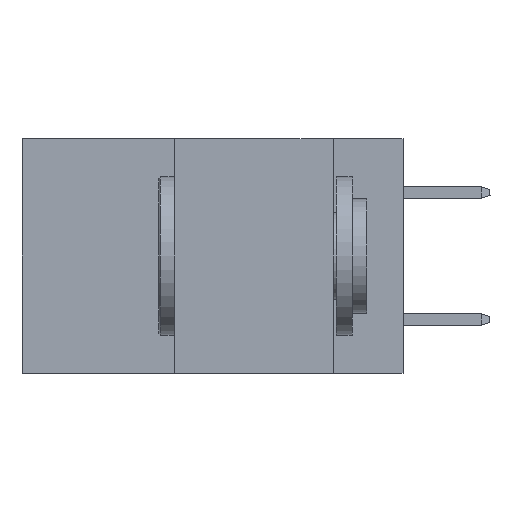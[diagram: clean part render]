
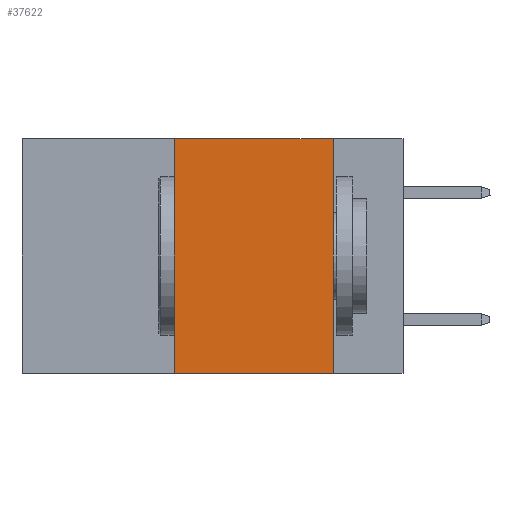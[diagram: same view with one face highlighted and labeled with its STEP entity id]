
A CAD part, left-side view. The second image highlights one B-rep face of the part: STEP entity #37622.
In plain terms, the highlighted planar face has unit normal (-1, 0, 0).
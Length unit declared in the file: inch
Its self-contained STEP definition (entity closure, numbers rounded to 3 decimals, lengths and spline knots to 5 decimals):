
#845 = DIRECTION ( 'NONE',  ( 0., -1., 0. ) ) ;
#2104 = ORIENTED_EDGE ( 'NONE', *, *, #20912, .T. ) ;
#2998 = CARTESIAN_POINT ( 'NONE',  ( 0., 0.36, 0. ) ) ;
#3638 = ORIENTED_EDGE ( 'NONE', *, *, #14503, .F. ) ;
#3734 = VERTEX_POINT ( 'NONE', #7135 ) ;
#6208 = ORIENTED_EDGE ( 'NONE', *, *, #8714, .F. ) ;
#7029 = EDGE_CURVE ( 'NONE', #15164, #10686, #27835, .T. ) ;
#7135 = CARTESIAN_POINT ( 'NONE',  ( 0., 0.36, 0. ) ) ;
#8320 = VERTEX_POINT ( 'NONE', #39944 ) ;
#8714 = EDGE_CURVE ( 'NONE', #3734, #15164, #33091, .T. ) ;
#10686 = VERTEX_POINT ( 'NONE', #17013 ) ;
#11775 = AXIS2_PLACEMENT_3D ( 'NONE', #17467, #36480, #36876 ) ;
#14037 = VECTOR ( 'NONE', #16190, 39.37008 ) ;
#14187 = VECTOR ( 'NONE', #845, 39.37008 ) ;
#14503 = EDGE_CURVE ( 'NONE', #8320, #3734, #33651, .T. ) ;
#15164 = VERTEX_POINT ( 'NONE', #24158 ) ;
#16190 = DIRECTION ( 'NONE',  ( 0., -1., 0. ) ) ;
#16596 = CARTESIAN_POINT ( 'NONE',  ( 0., 0.6, 0. ) ) ;
#16894 = VECTOR ( 'NONE', #30778, 39.37008 ) ;
#17013 = CARTESIAN_POINT ( 'NONE',  ( 0., 0.11, -0.37 ) ) ;
#17467 = CARTESIAN_POINT ( 'NONE',  ( 0., 0.6, 0. ) ) ;
#17676 = FACE_OUTER_BOUND ( 'NONE', #38625, .T. ) ;
#20912 = EDGE_CURVE ( 'NONE', #8320, #10686, #28253, .T. ) ;
#22736 = ORIENTED_EDGE ( 'NONE', *, *, #7029, .F. ) ;
#24158 = CARTESIAN_POINT ( 'NONE',  ( 0., 0.11, 0. ) ) ;
#25575 = CARTESIAN_POINT ( 'NONE',  ( 0., 0.6, -0.37 ) ) ;
#27835 = LINE ( 'NONE', #33327, #29616 ) ;
#28253 = LINE ( 'NONE', #25575, #14187 ) ;
#29616 = VECTOR ( 'NONE', #39890, 39.37008 ) ;
#30778 = DIRECTION ( 'NONE',  ( 0., 0., 1. ) ) ;
#33091 = LINE ( 'NONE', #16596, #14037 ) ;
#33327 = CARTESIAN_POINT ( 'NONE',  ( 0., 0.11, 0. ) ) ;
#33651 = LINE ( 'NONE', #2998, #16894 ) ;
#36480 = DIRECTION ( 'NONE',  ( 1., 0., 0. ) ) ;
#36876 = DIRECTION ( 'NONE',  ( 0., 0., -1. ) ) ;
#37622 = ADVANCED_FACE ( 'NONE', ( #17676 ), #39748, .F. ) ;
#38625 = EDGE_LOOP ( 'NONE', ( #22736, #6208, #3638, #2104 ) ) ;
#39748 = PLANE ( 'NONE',  #11775 ) ;
#39890 = DIRECTION ( 'NONE',  ( 0., 0., -1. ) ) ;
#39944 = CARTESIAN_POINT ( 'NONE',  ( 0., 0.36, -0.37 ) ) ;
